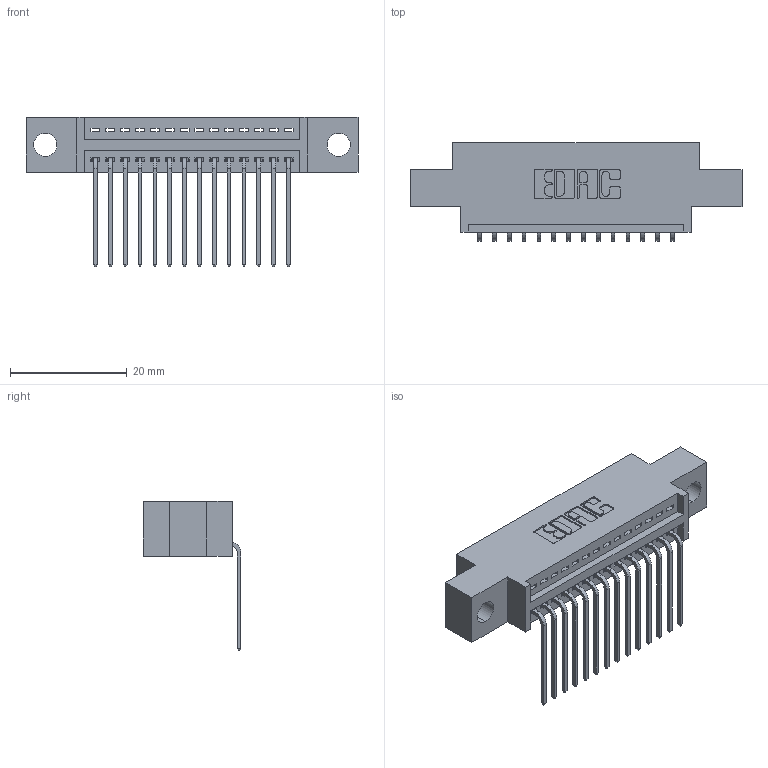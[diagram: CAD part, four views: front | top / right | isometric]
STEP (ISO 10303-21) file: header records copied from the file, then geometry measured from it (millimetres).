
FILE_DESCRIPTION (( 'STEP AP203' ), '1' );
FILE_NAME ('395-014-559-604.STEP', '2018-11-06T12:10:50', ( '' ), ( '' ), 'SwSTEP 2.0', 'SolidWorks 2016', '' );
FILE_SCHEMA (( 'CONFIG_CONTROL_DESIGN' ));
Length unit declared in the file: inch
Products named in the file (3): 395-014-559-604; 345-292-001_558 559 Tail - 1; 345 Part_0.170 Offset - 0.156 Dia-TH
Assembly tree (15 placements, depth 2):
  395-014-559-604
    345 Part_0.170 Offset - 0.156 Dia-TH
    345-292-001_558 559 Tail - 1  x14
Bounding box: 56.77 x 16.75 x 25.53 mm (x, y, z)
Volume: 5008 mm3; surface area: 6484 mm2
Topology: 15 solids, 15 shells, 970 faces, 2901 edges, 1914 vertices
Faces by surface type: plane 672, cylinder 298
Entity records: 14525 total; most frequent: CARTESIAN_POINT 2526, ORIENTED_EDGE 2474, DIRECTION 2245, EDGE_CURVE 1237, VECTOR 1049, LINE 1049, VERTEX_POINT 822, AXIS2_PLACEMENT_3D 598
